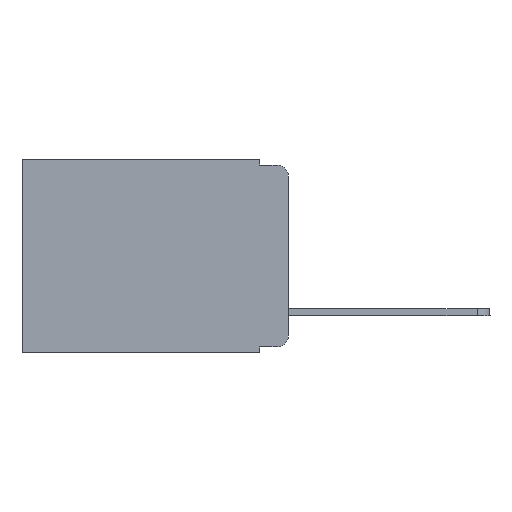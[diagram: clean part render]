
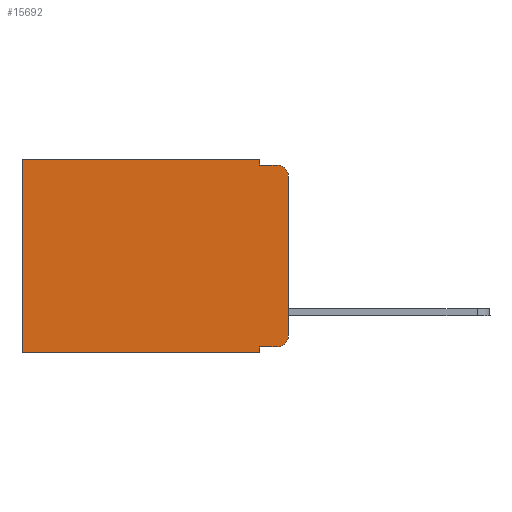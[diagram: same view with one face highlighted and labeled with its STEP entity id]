
A CAD part, left-side view. The second image highlights one B-rep face of the part: STEP entity #15692.
In plain terms, the highlighted planar face has unit normal (-1, 0, 0).
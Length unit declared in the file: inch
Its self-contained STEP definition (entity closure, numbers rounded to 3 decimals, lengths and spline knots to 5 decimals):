
#369 = LINE ( 'NONE', #9838, #1181 ) ;
#760 = AXIS2_PLACEMENT_3D ( 'NONE', #8589, #14041, #16529 ) ;
#783 = VERTEX_POINT ( 'NONE', #17412 ) ;
#1181 = VECTOR ( 'NONE', #13093, 39.37008 ) ;
#1412 = ORIENTED_EDGE ( 'NONE', *, *, #10411, .T. ) ;
#1591 = ORIENTED_EDGE ( 'NONE', *, *, #18563, .T. ) ;
#1811 = ORIENTED_EDGE ( 'NONE', *, *, #4670, .T. ) ;
#2186 = EDGE_CURVE ( 'NONE', #17656, #17388, #19279, .T. ) ;
#2263 = CARTESIAN_POINT ( 'NONE',  ( 0.298, 0.02, -0.313 ) ) ;
#2623 = VECTOR ( 'NONE', #8291, 39.37008 ) ;
#2825 = VECTOR ( 'NONE', #4928, 39.37008 ) ;
#2853 = ORIENTED_EDGE ( 'NONE', *, *, #20903, .F. ) ;
#2889 = VECTOR ( 'NONE', #5688, 39.37008 ) ;
#3028 = DIRECTION ( 'NONE',  ( 0., 0., -1. ) ) ;
#3801 = VERTEX_POINT ( 'NONE', #16402 ) ;
#3935 = DIRECTION ( 'NONE',  ( -1., 0., 0. ) ) ;
#3947 = ORIENTED_EDGE ( 'NONE', *, *, #15460, .F. ) ;
#4231 = DIRECTION ( 'NONE',  ( 0., -1., 0. ) ) ;
#4260 = DIRECTION ( 'NONE',  ( 0., 0., -1. ) ) ;
#4670 = EDGE_CURVE ( 'NONE', #10624, #12589, #6162, .T. ) ;
#4928 = DIRECTION ( 'NONE',  ( 0., 0., -1. ) ) ;
#5053 = AXIS2_PLACEMENT_3D ( 'NONE', #2263, #3935, #4260 ) ;
#5688 = DIRECTION ( 'NONE',  ( 0., 0., -1. ) ) ;
#6162 = LINE ( 'NONE', #11151, #18639 ) ;
#6178 = VERTEX_POINT ( 'NONE', #15199 ) ;
#7086 = EDGE_LOOP ( 'NONE', ( #2853, #14067, #9209, #3947, #1811, #1591, #9200, #7747, #11375, #1412 ) ) ;
#7379 = CIRCLE ( 'NONE', #14730, 0.02 ) ;
#7435 = LINE ( 'NONE', #22216, #2825 ) ;
#7639 = CARTESIAN_POINT ( 'NONE',  ( 0.298, 0.051, -0.333 ) ) ;
#7747 = ORIENTED_EDGE ( 'NONE', *, *, #22295, .F. ) ;
#8192 = DIRECTION ( 'NONE',  ( -1., 0., 0. ) ) ;
#8291 = DIRECTION ( 'NONE',  ( 0., 0., -1. ) ) ;
#8587 = CARTESIAN_POINT ( 'NONE',  ( 0.298, 0.051, 0. ) ) ;
#8589 = CARTESIAN_POINT ( 'NONE',  ( 0.298, 0., 0. ) ) ;
#8743 = VERTEX_POINT ( 'NONE', #16254 ) ;
#8771 = PLANE ( 'NONE',  #760 ) ;
#8897 = VECTOR ( 'NONE', #4231, 39.37008 ) ;
#8953 = EDGE_CURVE ( 'NONE', #6178, #3801, #7379, .T. ) ;
#9144 = CARTESIAN_POINT ( 'NONE',  ( 0.298, 0.473, -0.343 ) ) ;
#9200 = ORIENTED_EDGE ( 'NONE', *, *, #2186, .F. ) ;
#9209 = ORIENTED_EDGE ( 'NONE', *, *, #21705, .F. ) ;
#9838 = CARTESIAN_POINT ( 'NONE',  ( 0.298, 0.051, -0.01 ) ) ;
#10411 = EDGE_CURVE ( 'NONE', #14754, #783, #22489, .T. ) ;
#10624 = VERTEX_POINT ( 'NONE', #21712 ) ;
#10668 = CARTESIAN_POINT ( 'NONE',  ( 0.298, 0.02, -0.333 ) ) ;
#11095 = EDGE_CURVE ( 'NONE', #8743, #14754, #11882, .T. ) ;
#11151 = CARTESIAN_POINT ( 'NONE',  ( 0.298, 0., 0. ) ) ;
#11153 = VECTOR ( 'NONE', #15169, 39.37008 ) ;
#11312 = DIRECTION ( 'NONE',  ( 0., 1., 0. ) ) ;
#11375 = ORIENTED_EDGE ( 'NONE', *, *, #11095, .T. ) ;
#11882 = LINE ( 'NONE', #7639, #8897 ) ;
#12589 = VERTEX_POINT ( 'NONE', #14457 ) ;
#12907 = FACE_OUTER_BOUND ( 'NONE', #7086, .T. ) ;
#13093 = DIRECTION ( 'NONE',  ( 0., -1., 0. ) ) ;
#13954 = LINE ( 'NONE', #8587, #2623 ) ;
#14041 = DIRECTION ( 'NONE',  ( 1., 0., 0. ) ) ;
#14067 = ORIENTED_EDGE ( 'NONE', *, *, #8953, .T. ) ;
#14457 = CARTESIAN_POINT ( 'NONE',  ( 0.298, 0.473, 0. ) ) ;
#14730 = AXIS2_PLACEMENT_3D ( 'NONE', #15080, #8192, #3028 ) ;
#14754 = VERTEX_POINT ( 'NONE', #10668 ) ;
#15080 = CARTESIAN_POINT ( 'NONE',  ( 0.298, 0.02, -0.03 ) ) ;
#15169 = DIRECTION ( 'NONE',  ( 0., 1., 0. ) ) ;
#15199 = CARTESIAN_POINT ( 'NONE',  ( 0.298, 0., -0.03 ) ) ;
#15460 = EDGE_CURVE ( 'NONE', #10624, #17862, #13954, .T. ) ;
#15692 = ADVANCED_FACE ( 'NONE', ( #12907 ), #8771, .F. ) ;
#16254 = CARTESIAN_POINT ( 'NONE',  ( 0.298, 0.051, -0.333 ) ) ;
#16402 = CARTESIAN_POINT ( 'NONE',  ( 0.298, 0.02, -0.01 ) ) ;
#16529 = DIRECTION ( 'NONE',  ( 0., 0., -1. ) ) ;
#16831 = LINE ( 'NONE', #20991, #17366 ) ;
#17366 = VECTOR ( 'NONE', #19019, 39.37008 ) ;
#17388 = VERTEX_POINT ( 'NONE', #9144 ) ;
#17412 = CARTESIAN_POINT ( 'NONE',  ( 0.298, 0., -0.313 ) ) ;
#17656 = VERTEX_POINT ( 'NONE', #21655 ) ;
#17862 = VERTEX_POINT ( 'NONE', #18390 ) ;
#18390 = CARTESIAN_POINT ( 'NONE',  ( 0.298, 0.051, -0.01 ) ) ;
#18563 = EDGE_CURVE ( 'NONE', #12589, #17388, #16831, .T. ) ;
#18639 = VECTOR ( 'NONE', #11312, 39.37008 ) ;
#19019 = DIRECTION ( 'NONE',  ( 0., 0., -1. ) ) ;
#19279 = LINE ( 'NONE', #22096, #11153 ) ;
#20903 = EDGE_CURVE ( 'NONE', #6178, #783, #21069, .T. ) ;
#20991 = CARTESIAN_POINT ( 'NONE',  ( 0.298, 0.473, 0. ) ) ;
#21069 = LINE ( 'NONE', #21080, #2889 ) ;
#21080 = CARTESIAN_POINT ( 'NONE',  ( 0.298, 0., 0. ) ) ;
#21655 = CARTESIAN_POINT ( 'NONE',  ( 0.298, 0.051, -0.343 ) ) ;
#21705 = EDGE_CURVE ( 'NONE', #17862, #3801, #369, .T. ) ;
#21712 = CARTESIAN_POINT ( 'NONE',  ( 0.298, 0.051, 0. ) ) ;
#22096 = CARTESIAN_POINT ( 'NONE',  ( 0.298, 0., -0.343 ) ) ;
#22216 = CARTESIAN_POINT ( 'NONE',  ( 0.298, 0.051, 0. ) ) ;
#22295 = EDGE_CURVE ( 'NONE', #8743, #17656, #7435, .T. ) ;
#22489 = CIRCLE ( 'NONE', #5053, 0.02 ) ;
